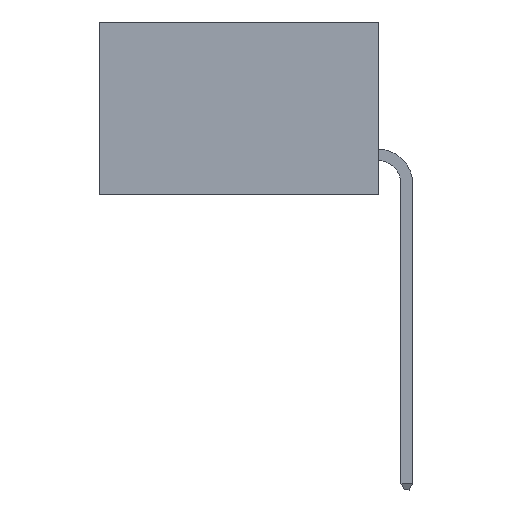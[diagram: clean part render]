
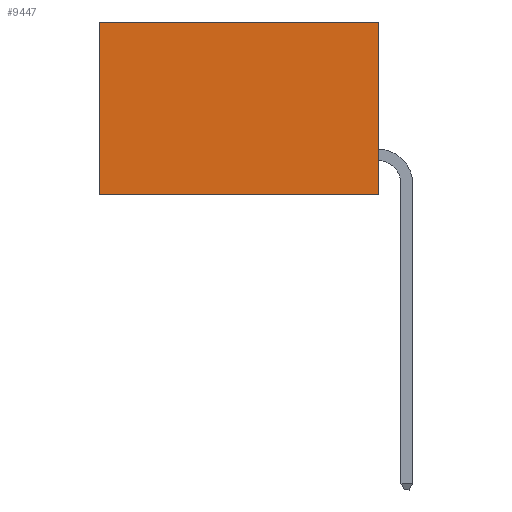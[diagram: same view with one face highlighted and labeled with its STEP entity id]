
A CAD part, left-side view. The second image highlights one B-rep face of the part: STEP entity #9447.
In plain terms, the highlighted planar face has unit normal (-1, 0, 0).
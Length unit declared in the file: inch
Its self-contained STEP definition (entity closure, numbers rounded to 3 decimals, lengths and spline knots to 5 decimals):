
#177 = CARTESIAN_POINT ( 'NONE',  ( 0.298, 0., 0. ) ) ;
#492 = VERTEX_POINT ( 'NONE', #6717 ) ;
#1479 = LINE ( 'NONE', #10163, #9666 ) ;
#1887 = EDGE_CURVE ( 'NONE', #17855, #6964, #20986, .T. ) ;
#2353 = ORIENTED_EDGE ( 'NONE', *, *, #10125, .T. ) ;
#2468 = DIRECTION ( 'NONE',  ( 0., 1., 0. ) ) ;
#2587 = EDGE_CURVE ( 'NONE', #10702, #492, #15446, .T. ) ;
#2814 = LINE ( 'NONE', #5733, #10975 ) ;
#3176 = AXIS2_PLACEMENT_3D ( 'NONE', #13608, #4017, #4378 ) ;
#4017 = DIRECTION ( 'NONE',  ( 1., 0., 0. ) ) ;
#4378 = DIRECTION ( 'NONE',  ( 0., 0., -1. ) ) ;
#5733 = CARTESIAN_POINT ( 'NONE',  ( 0.298, 0., -0.37 ) ) ;
#6717 = CARTESIAN_POINT ( 'NONE',  ( 0.298, 0.6, -0.37 ) ) ;
#6856 = ORIENTED_EDGE ( 'NONE', *, *, #9441, .F. ) ;
#6964 = VERTEX_POINT ( 'NONE', #16017 ) ;
#9441 = EDGE_CURVE ( 'NONE', #6964, #492, #2814, .T. ) ;
#9447 = ADVANCED_FACE ( 'NONE', ( #14860 ), #13632, .F. ) ;
#9666 = VECTOR ( 'NONE', #2468, 39.37008 ) ;
#10125 = EDGE_CURVE ( 'NONE', #17855, #10702, #1479, .T. ) ;
#10163 = CARTESIAN_POINT ( 'NONE',  ( 0.298, 0., 0. ) ) ;
#10702 = VERTEX_POINT ( 'NONE', #17520 ) ;
#10975 = VECTOR ( 'NONE', #13452, 39.37008 ) ;
#11042 = VECTOR ( 'NONE', #15479, 39.37008 ) ;
#11882 = ORIENTED_EDGE ( 'NONE', *, *, #2587, .T. ) ;
#12994 = EDGE_LOOP ( 'NONE', ( #11882, #6856, #15316, #2353 ) ) ;
#13452 = DIRECTION ( 'NONE',  ( 0., 1., 0. ) ) ;
#13608 = CARTESIAN_POINT ( 'NONE',  ( 0.298, 0., 0. ) ) ;
#13632 = PLANE ( 'NONE',  #3176 ) ;
#14232 = DIRECTION ( 'NONE',  ( 0., 0., -1. ) ) ;
#14860 = FACE_OUTER_BOUND ( 'NONE', #12994, .T. ) ;
#15260 = CARTESIAN_POINT ( 'NONE',  ( 0.298, 0.6, 0. ) ) ;
#15316 = ORIENTED_EDGE ( 'NONE', *, *, #1887, .F. ) ;
#15446 = LINE ( 'NONE', #15260, #11042 ) ;
#15479 = DIRECTION ( 'NONE',  ( 0., 0., -1. ) ) ;
#16017 = CARTESIAN_POINT ( 'NONE',  ( 0.298, 0., -0.37 ) ) ;
#17232 = VECTOR ( 'NONE', #14232, 39.37008 ) ;
#17520 = CARTESIAN_POINT ( 'NONE',  ( 0.298, 0.6, 0. ) ) ;
#17855 = VERTEX_POINT ( 'NONE', #21149 ) ;
#20986 = LINE ( 'NONE', #177, #17232 ) ;
#21149 = CARTESIAN_POINT ( 'NONE',  ( 0.298, 0., 0. ) ) ;
